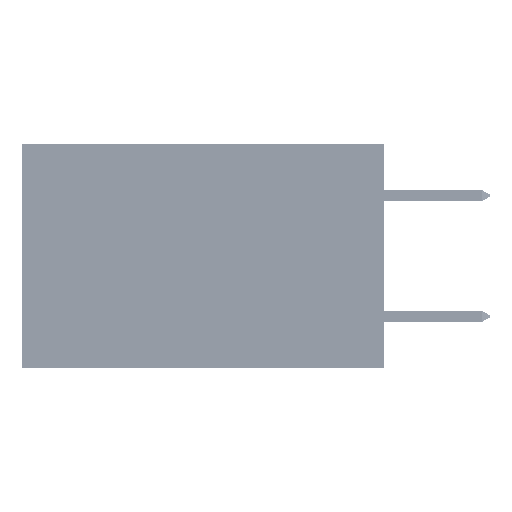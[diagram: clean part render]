
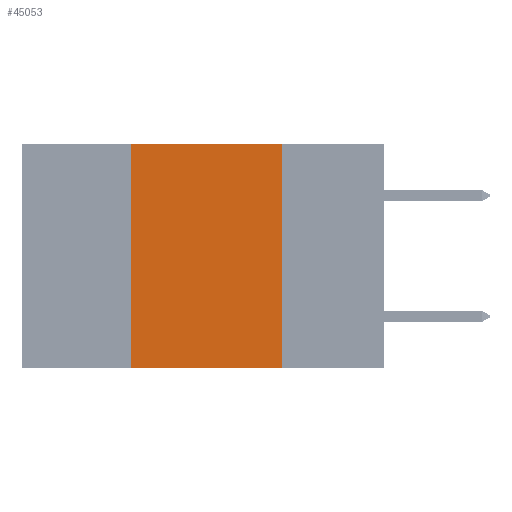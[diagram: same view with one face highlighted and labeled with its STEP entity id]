
A CAD part, left-side view. The second image highlights one B-rep face of the part: STEP entity #45053.
In plain terms, the highlighted planar face has unit normal (-1, 0, 0).
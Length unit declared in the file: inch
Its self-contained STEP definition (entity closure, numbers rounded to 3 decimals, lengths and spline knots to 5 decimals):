
#799 = DIRECTION ( 'NONE',  ( 0., 0., -1. ) ) ;
#1112 = CARTESIAN_POINT ( 'NONE',  ( 0., 0.6, 0. ) ) ;
#1587 = ORIENTED_EDGE ( 'NONE', *, *, #14386, .F. ) ;
#2030 = ORIENTED_EDGE ( 'NONE', *, *, #13848, .T. ) ;
#4262 = VECTOR ( 'NONE', #17223, 39.37008 ) ;
#6038 = VECTOR ( 'NONE', #46477, 39.37008 ) ;
#6278 = VERTEX_POINT ( 'NONE', #31005 ) ;
#6826 = CARTESIAN_POINT ( 'NONE',  ( 0., 0.6, -0.37 ) ) ;
#7030 = EDGE_CURVE ( 'NONE', #6278, #20079, #11744, .T. ) ;
#9820 = LINE ( 'NONE', #28840, #29650 ) ;
#9897 = AXIS2_PLACEMENT_3D ( 'NONE', #1112, #22413, #799 ) ;
#11744 = LINE ( 'NONE', #37076, #39474 ) ;
#13848 = EDGE_CURVE ( 'NONE', #36576, #19927, #15636, .T. ) ;
#14386 = EDGE_CURVE ( 'NONE', #36576, #6278, #21181, .T. ) ;
#14854 = PLANE ( 'NONE',  #9897 ) ;
#15421 = DIRECTION ( 'NONE',  ( 0., -1., 0. ) ) ;
#15636 = LINE ( 'NONE', #6826, #6038 ) ;
#17075 = EDGE_LOOP ( 'NONE', ( #36557, #22682, #1587, #2030 ) ) ;
#17223 = DIRECTION ( 'NONE',  ( 0., 0., 1. ) ) ;
#18387 = CARTESIAN_POINT ( 'NONE',  ( 0., 0.17, -0.37 ) ) ;
#19927 = VERTEX_POINT ( 'NONE', #18387 ) ;
#20079 = VERTEX_POINT ( 'NONE', #33566 ) ;
#20085 = CARTESIAN_POINT ( 'NONE',  ( 0., 0.42, -0.37 ) ) ;
#21181 = LINE ( 'NONE', #35546, #4262 ) ;
#22413 = DIRECTION ( 'NONE',  ( 1., 0., 0. ) ) ;
#22682 = ORIENTED_EDGE ( 'NONE', *, *, #7030, .F. ) ;
#24302 = FACE_OUTER_BOUND ( 'NONE', #17075, .T. ) ;
#28840 = CARTESIAN_POINT ( 'NONE',  ( 0., 0.17, 0. ) ) ;
#29650 = VECTOR ( 'NONE', #40228, 39.37008 ) ;
#31005 = CARTESIAN_POINT ( 'NONE',  ( 0., 0.42, 0. ) ) ;
#33566 = CARTESIAN_POINT ( 'NONE',  ( 0., 0.17, 0. ) ) ;
#35546 = CARTESIAN_POINT ( 'NONE',  ( 0., 0.42, 0. ) ) ;
#36557 = ORIENTED_EDGE ( 'NONE', *, *, #42833, .F. ) ;
#36576 = VERTEX_POINT ( 'NONE', #20085 ) ;
#37076 = CARTESIAN_POINT ( 'NONE',  ( 0., 0.6, 0. ) ) ;
#39474 = VECTOR ( 'NONE', #15421, 39.37008 ) ;
#40228 = DIRECTION ( 'NONE',  ( 0., 0., -1. ) ) ;
#42833 = EDGE_CURVE ( 'NONE', #20079, #19927, #9820, .T. ) ;
#45053 = ADVANCED_FACE ( 'NONE', ( #24302 ), #14854, .F. ) ;
#46477 = DIRECTION ( 'NONE',  ( 0., -1., 0. ) ) ;
